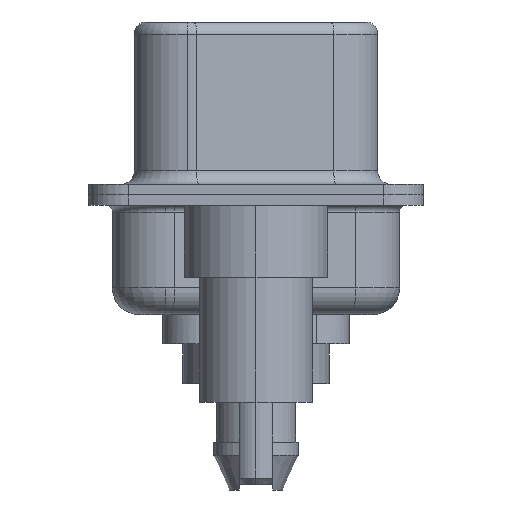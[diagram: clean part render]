
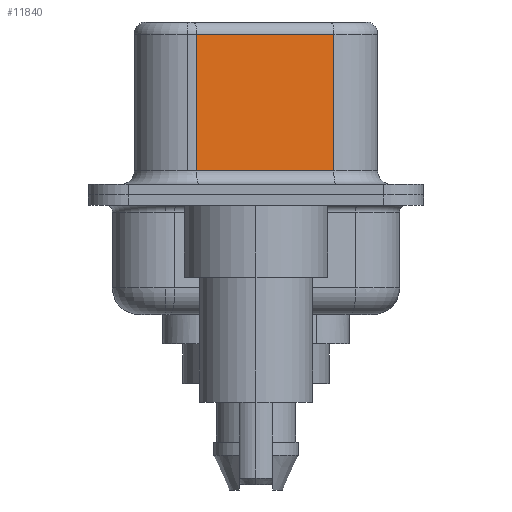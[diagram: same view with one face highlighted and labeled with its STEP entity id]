
A CAD part, left-side view. The second image highlights one B-rep face of the part: STEP entity #11840.
In plain terms, the highlighted planar face has unit normal (-0.985, -0.174, 0).
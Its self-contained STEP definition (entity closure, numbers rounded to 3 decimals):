
#358 = ORIENTED_EDGE ( 'NONE', *, *, #2067, .T. ) ;
#698 = ORIENTED_EDGE ( 'NONE', *, *, #17915, .T. ) ;
#875 = CARTESIAN_POINT ( 'NONE',  ( 3.675, 2.233, 6.52 ) ) ;
#1656 = CARTESIAN_POINT ( 'NONE',  ( 4.585, -2.927, 6.52 ) ) ;
#2067 = EDGE_CURVE ( 'NONE', #16610, #16304, #17379, .T. ) ;
#2597 = LINE ( 'NONE', #11351, #10506 ) ;
#3316 = CARTESIAN_POINT ( 'NONE',  ( 3.675, 2.233, 0.9 ) ) ;
#3485 = VECTOR ( 'NONE', #12851, 1000. ) ;
#3603 = CARTESIAN_POINT ( 'NONE',  ( 4.585, -2.927, 0.9 ) ) ;
#4060 = CARTESIAN_POINT ( 'NONE',  ( 4.585, -2.927, 6.02 ) ) ;
#4683 = DIRECTION ( 'NONE',  ( 0.985, 0.174, 0. ) ) ;
#5054 = CARTESIAN_POINT ( 'NONE',  ( 3.675, 2.233, 6.02 ) ) ;
#7579 = EDGE_LOOP ( 'NONE', ( #13044, #358, #698, #19076 ) ) ;
#8329 = EDGE_CURVE ( 'NONE', #16877, #12810, #14775, .T. ) ;
#9266 = FACE_OUTER_BOUND ( 'NONE', #7579, .T. ) ;
#10317 = VECTOR ( 'NONE', #18513, 1000. ) ;
#10324 = AXIS2_PLACEMENT_3D ( 'NONE', #1656, #4683, #15122 ) ;
#10506 = VECTOR ( 'NONE', #18849, 1000. ) ;
#11351 = CARTESIAN_POINT ( 'NONE',  ( 4.585, -2.927, 6.52 ) ) ;
#11552 = CARTESIAN_POINT ( 'NONE',  ( 4.585, -2.927, 6.02 ) ) ;
#11840 = ADVANCED_FACE ( 'NONE', ( #9266 ), #18082, .F. ) ;
#12810 = VERTEX_POINT ( 'NONE', #17368 ) ;
#12851 = DIRECTION ( 'NONE',  ( 0., 0., -1. ) ) ;
#13044 = ORIENTED_EDGE ( 'NONE', *, *, #15335, .F. ) ;
#14775 = LINE ( 'NONE', #3603, #10317 ) ;
#14929 = LINE ( 'NONE', #875, #3485 ) ;
#15122 = DIRECTION ( 'NONE',  ( -0.174, 0.985, 0. ) ) ;
#15335 = EDGE_CURVE ( 'NONE', #16610, #12810, #2597, .T. ) ;
#16304 = VERTEX_POINT ( 'NONE', #5054 ) ;
#16610 = VERTEX_POINT ( 'NONE', #4060 ) ;
#16877 = VERTEX_POINT ( 'NONE', #3316 ) ;
#16910 = VECTOR ( 'NONE', #18067, 1000. ) ;
#17368 = CARTESIAN_POINT ( 'NONE',  ( 4.585, -2.927, 0.9 ) ) ;
#17379 = LINE ( 'NONE', #11552, #16910 ) ;
#17915 = EDGE_CURVE ( 'NONE', #16304, #16877, #14929, .T. ) ;
#18067 = DIRECTION ( 'NONE',  ( -0.174, 0.985, 0. ) ) ;
#18082 = PLANE ( 'NONE',  #10324 ) ;
#18513 = DIRECTION ( 'NONE',  ( 0.174, -0.985, 0. ) ) ;
#18849 = DIRECTION ( 'NONE',  ( 0., 0., -1. ) ) ;
#19076 = ORIENTED_EDGE ( 'NONE', *, *, #8329, .T. ) ;
